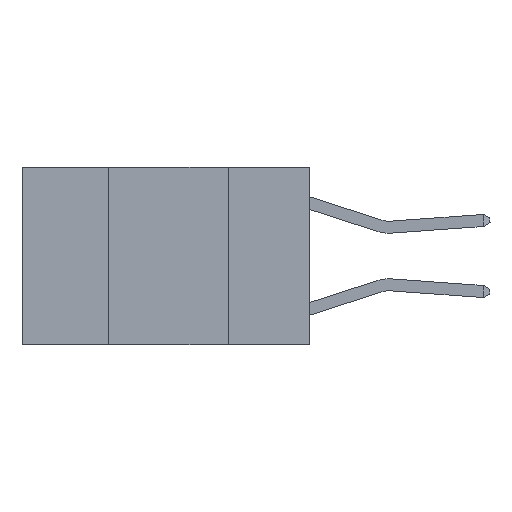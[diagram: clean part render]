
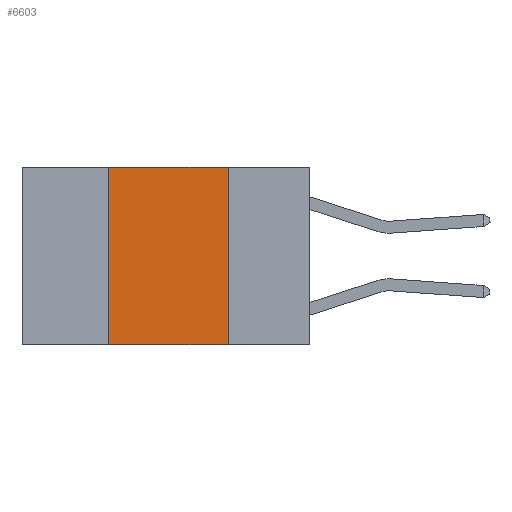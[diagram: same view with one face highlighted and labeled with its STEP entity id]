
A CAD part, left-side view. The second image highlights one B-rep face of the part: STEP entity #6603.
In plain terms, the highlighted planar face has unit normal (-1, 0, 0).
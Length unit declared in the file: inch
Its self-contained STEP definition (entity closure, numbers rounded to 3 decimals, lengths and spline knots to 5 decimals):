
#45 = CARTESIAN_POINT ( 'NONE',  ( 0., 0.6, -0.37 ) ) ;
#67 = VERTEX_POINT ( 'NONE', #8612 ) ;
#1076 = DIRECTION ( 'NONE',  ( 0., -1., 0. ) ) ;
#1768 = LINE ( 'NONE', #45, #6680 ) ;
#1909 = DIRECTION ( 'NONE',  ( 0., 0., 1. ) ) ;
#2147 = EDGE_CURVE ( 'NONE', #10359, #3992, #1768, .T. ) ;
#2798 = EDGE_CURVE ( 'NONE', #7739, #67, #11341, .T. ) ;
#3120 = LINE ( 'NONE', #8713, #8545 ) ;
#3191 = DIRECTION ( 'NONE',  ( 1., 0., 0. ) ) ;
#3984 = CARTESIAN_POINT ( 'NONE',  ( 0., 0.17, 0. ) ) ;
#3992 = VERTEX_POINT ( 'NONE', #4929 ) ;
#4604 = CARTESIAN_POINT ( 'NONE',  ( 0., 0.6, 0. ) ) ;
#4696 = CARTESIAN_POINT ( 'NONE',  ( 0., 0.42, -0.37 ) ) ;
#4722 = AXIS2_PLACEMENT_3D ( 'NONE', #6102, #3191, #9934 ) ;
#4929 = CARTESIAN_POINT ( 'NONE',  ( 0., 0.17, -0.37 ) ) ;
#5130 = VECTOR ( 'NONE', #6880, 39.37008 ) ;
#5680 = FACE_OUTER_BOUND ( 'NONE', #10199, .T. ) ;
#6102 = CARTESIAN_POINT ( 'NONE',  ( 0., 0.6, 0. ) ) ;
#6603 = ADVANCED_FACE ( 'NONE', ( #5680 ), #8978, .F. ) ;
#6656 = VECTOR ( 'NONE', #11154, 39.37008 ) ;
#6680 = VECTOR ( 'NONE', #1076, 39.37008 ) ;
#6880 = DIRECTION ( 'NONE',  ( 0., 0., -1. ) ) ;
#7196 = ORIENTED_EDGE ( 'NONE', *, *, #11629, .F. ) ;
#7497 = ORIENTED_EDGE ( 'NONE', *, *, #2147, .T. ) ;
#7739 = VERTEX_POINT ( 'NONE', #10338 ) ;
#8545 = VECTOR ( 'NONE', #1909, 39.37008 ) ;
#8612 = CARTESIAN_POINT ( 'NONE',  ( 0., 0.17, 0. ) ) ;
#8713 = CARTESIAN_POINT ( 'NONE',  ( 0., 0.42, 0. ) ) ;
#8849 = ORIENTED_EDGE ( 'NONE', *, *, #2798, .F. ) ;
#8978 = PLANE ( 'NONE',  #4722 ) ;
#9934 = DIRECTION ( 'NONE',  ( 0., 0., -1. ) ) ;
#10184 = LINE ( 'NONE', #3984, #5130 ) ;
#10199 = EDGE_LOOP ( 'NONE', ( #11021, #8849, #7196, #7497 ) ) ;
#10338 = CARTESIAN_POINT ( 'NONE',  ( 0., 0.42, 0. ) ) ;
#10359 = VERTEX_POINT ( 'NONE', #4696 ) ;
#11021 = ORIENTED_EDGE ( 'NONE', *, *, #11666, .F. ) ;
#11154 = DIRECTION ( 'NONE',  ( 0., -1., 0. ) ) ;
#11341 = LINE ( 'NONE', #4604, #6656 ) ;
#11629 = EDGE_CURVE ( 'NONE', #10359, #7739, #3120, .T. ) ;
#11666 = EDGE_CURVE ( 'NONE', #67, #3992, #10184, .T. ) ;
